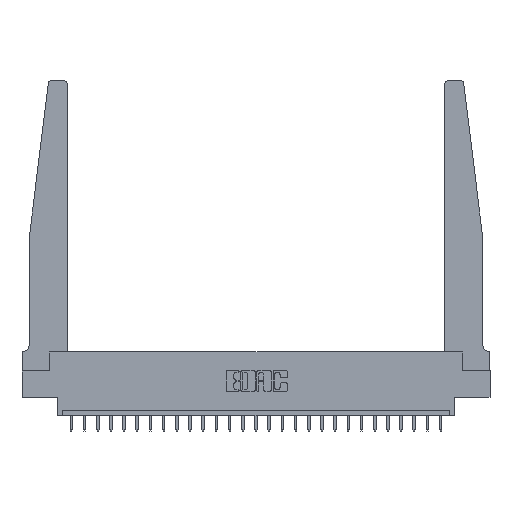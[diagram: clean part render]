
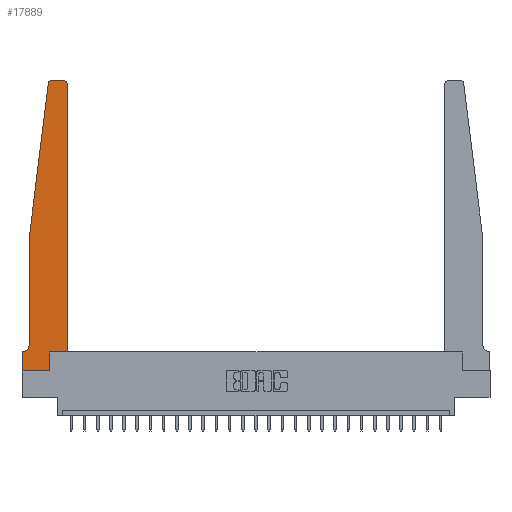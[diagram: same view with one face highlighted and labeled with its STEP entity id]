
A CAD part, top view. The second image highlights one B-rep face of the part: STEP entity #17889.
In plain terms, the highlighted planar face has unit normal (0, 0, 1).
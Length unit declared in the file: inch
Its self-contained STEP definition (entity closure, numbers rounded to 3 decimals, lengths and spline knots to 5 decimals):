
#10 = FACE_OUTER_BOUND ( 'NONE', #18840, .T. ) ;
#721 = DIRECTION ( 'NONE',  ( 0., -1., 0. ) ) ;
#957 = ORIENTED_EDGE ( 'NONE', *, *, #10690, .T. ) ;
#1084 = DIRECTION ( 'NONE',  ( 0., 1., 0. ) ) ;
#1565 = CARTESIAN_POINT ( 'NONE',  ( 0., 0.1875, 0.37 ) ) ;
#1606 = EDGE_CURVE ( 'NONE', #12865, #8407, #6839, .T. ) ;
#1644 = ORIENTED_EDGE ( 'NONE', *, *, #5036, .T. ) ;
#1809 = VERTEX_POINT ( 'NONE', #23196 ) ;
#2691 = ORIENTED_EDGE ( 'NONE', *, *, #24000, .T. ) ;
#2729 = DIRECTION ( 'NONE',  ( 0., 1., 0. ) ) ;
#2751 = VERTEX_POINT ( 'NONE', #13256 ) ;
#2815 = VERTEX_POINT ( 'NONE', #23662 ) ;
#3109 = ORIENTED_EDGE ( 'NONE', *, *, #23587, .T. ) ;
#3194 = VECTOR ( 'NONE', #2729, 39.37008 ) ;
#3248 = VERTEX_POINT ( 'NONE', #16357 ) ;
#3302 = AXIS2_PLACEMENT_3D ( 'NONE', #1565, #9700, #10102 ) ;
#3491 = AXIS2_PLACEMENT_3D ( 'NONE', #4339, #17725, #12045 ) ;
#3916 = ORIENTED_EDGE ( 'NONE', *, *, #8207, .T. ) ;
#3997 = VERTEX_POINT ( 'NONE', #21458 ) ;
#4089 = VERTEX_POINT ( 'NONE', #14762 ) ;
#4339 = CARTESIAN_POINT ( 'NONE',  ( 0.395, 2.72, 0.37 ) ) ;
#4904 = DIRECTION ( 'NONE',  ( 0., 0., -1. ) ) ;
#5036 = EDGE_CURVE ( 'NONE', #8407, #12965, #13755, .T. ) ;
#5824 = DIRECTION ( 'NONE',  ( 1., 0., 0. ) ) ;
#5901 = CARTESIAN_POINT ( 'NONE',  ( 0.27653, 2.72, 0.37 ) ) ;
#6569 = VECTOR ( 'NONE', #14403, 39.37008 ) ;
#6823 = DIRECTION ( 'NONE',  ( -1., 0., 0. ) ) ;
#6839 = CIRCLE ( 'NONE', #8254, 0.05 ) ;
#7009 = EDGE_CURVE ( 'NONE', #24431, #12865, #10088, .T. ) ;
#7024 = VECTOR ( 'NONE', #9410, 39.37008 ) ;
#7261 = VECTOR ( 'NONE', #1084, 39.37008 ) ;
#7342 = VERTEX_POINT ( 'NONE', #7566 ) ;
#7566 = CARTESIAN_POINT ( 'NONE',  ( 0., 0., 0.37 ) ) ;
#7690 = ORIENTED_EDGE ( 'NONE', *, *, #12557, .T. ) ;
#8207 = EDGE_CURVE ( 'NONE', #7342, #3248, #18680, .T. ) ;
#8254 = AXIS2_PLACEMENT_3D ( 'NONE', #16373, #4904, #6823 ) ;
#8407 = VERTEX_POINT ( 'NONE', #11729 ) ;
#8481 = LINE ( 'NONE', #8640, #7261 ) ;
#8640 = CARTESIAN_POINT ( 'NONE',  ( 0.2605, 0.18, 0.37 ) ) ;
#8898 = LINE ( 'NONE', #21751, #3194 ) ;
#9410 = DIRECTION ( 'NONE',  ( 1., 0., 0. ) ) ;
#9700 = DIRECTION ( 'NONE',  ( 0., 0., 1. ) ) ;
#9701 = VECTOR ( 'NONE', #11480, 39.37008 ) ;
#10005 = VECTOR ( 'NONE', #721, 39.37008 ) ;
#10060 = CIRCLE ( 'NONE', #15033, 0.03 ) ;
#10088 = LINE ( 'NONE', #23839, #14315 ) ;
#10102 = DIRECTION ( 'NONE',  ( 1., 0., 0. ) ) ;
#10339 = VECTOR ( 'NONE', #17485, 39.37008 ) ;
#10530 = EDGE_CURVE ( 'NONE', #1809, #2815, #8898, .T. ) ;
#10690 = EDGE_CURVE ( 'NONE', #3997, #23022, #14297, .T. ) ;
#11480 = DIRECTION ( 'NONE',  ( -0.122, -0.992, 0. ) ) ;
#11729 = CARTESIAN_POINT ( 'NONE',  ( 0.015, 0.1875, 0.37 ) ) ;
#11876 = CARTESIAN_POINT ( 'NONE',  ( 0.425, 0.18, 0.37 ) ) ;
#12045 = DIRECTION ( 'NONE',  ( 1., 0., 0. ) ) ;
#12557 = EDGE_CURVE ( 'NONE', #3248, #4089, #8481, .T. ) ;
#12865 = VERTEX_POINT ( 'NONE', #16001 ) ;
#12965 = VERTEX_POINT ( 'NONE', #21461 ) ;
#13154 = ORIENTED_EDGE ( 'NONE', *, *, #1606, .T. ) ;
#13256 = CARTESIAN_POINT ( 'NONE',  ( 0.24675, 2.72367, 0.37 ) ) ;
#13571 = LINE ( 'NONE', #21082, #9701 ) ;
#13755 = LINE ( 'NONE', #20115, #6569 ) ;
#14296 = CARTESIAN_POINT ( 'NONE',  ( 0., 0., 0.37 ) ) ;
#14297 = LINE ( 'NONE', #14437, #17247 ) ;
#14315 = VECTOR ( 'NONE', #19960, 39.37008 ) ;
#14403 = DIRECTION ( 'NONE',  ( -1., 0., 0. ) ) ;
#14437 = CARTESIAN_POINT ( 'NONE',  ( 0.25, 2.75, 0.37 ) ) ;
#14762 = CARTESIAN_POINT ( 'NONE',  ( 0.2605, 0.18, 0.37 ) ) ;
#15033 = AXIS2_PLACEMENT_3D ( 'NONE', #5901, #17303, #5824 ) ;
#15222 = ORIENTED_EDGE ( 'NONE', *, *, #19550, .T. ) ;
#15533 = EDGE_CURVE ( 'NONE', #2815, #3997, #17134, .T. ) ;
#16001 = CARTESIAN_POINT ( 'NONE',  ( 0.065, 0.2375, 0.37 ) ) ;
#16251 = ORIENTED_EDGE ( 'NONE', *, *, #20805, .T. ) ;
#16357 = CARTESIAN_POINT ( 'NONE',  ( 0.2605, 0., 0.37 ) ) ;
#16373 = CARTESIAN_POINT ( 'NONE',  ( 0.015, 0.2375, 0.37 ) ) ;
#16885 = LINE ( 'NONE', #14296, #10005 ) ;
#16929 = CARTESIAN_POINT ( 'NONE',  ( 0., 0., 0.37 ) ) ;
#17134 = CIRCLE ( 'NONE', #3491, 0.03 ) ;
#17247 = VECTOR ( 'NONE', #22078, 39.37008 ) ;
#17303 = DIRECTION ( 'NONE',  ( 0., 0., 1. ) ) ;
#17485 = DIRECTION ( 'NONE',  ( 1., 0., 0. ) ) ;
#17656 = CARTESIAN_POINT ( 'NONE',  ( 0.27653, 2.75, 0.37 ) ) ;
#17725 = DIRECTION ( 'NONE',  ( 0., 0., 1. ) ) ;
#17889 = ADVANCED_FACE ( 'NONE', ( #10 ), #23643, .T. ) ;
#18335 = ORIENTED_EDGE ( 'NONE', *, *, #15533, .T. ) ;
#18346 = ORIENTED_EDGE ( 'NONE', *, *, #10530, .T. ) ;
#18680 = LINE ( 'NONE', #16929, #7024 ) ;
#18840 = EDGE_LOOP ( 'NONE', ( #957, #15222, #2691, #22019, #13154, #1644, #3109, #3916, #7690, #16251, #18346, #18335 ) ) ;
#19550 = EDGE_CURVE ( 'NONE', #23022, #2751, #10060, .T. ) ;
#19882 = LINE ( 'NONE', #11876, #10339 ) ;
#19960 = DIRECTION ( 'NONE',  ( 0., -1., 0. ) ) ;
#20115 = CARTESIAN_POINT ( 'NONE',  ( 0.065, 0.1875, 0.37 ) ) ;
#20805 = EDGE_CURVE ( 'NONE', #4089, #1809, #19882, .T. ) ;
#21082 = CARTESIAN_POINT ( 'NONE',  ( 0.065, 1.25, 0.37 ) ) ;
#21458 = CARTESIAN_POINT ( 'NONE',  ( 0.395, 2.75, 0.37 ) ) ;
#21461 = CARTESIAN_POINT ( 'NONE',  ( 0., 0.1875, 0.37 ) ) ;
#21478 = CARTESIAN_POINT ( 'NONE',  ( 0.065, 1.25, 0.37 ) ) ;
#21751 = CARTESIAN_POINT ( 'NONE',  ( 0.425, 0.18, 0.37 ) ) ;
#22019 = ORIENTED_EDGE ( 'NONE', *, *, #7009, .T. ) ;
#22078 = DIRECTION ( 'NONE',  ( -1., 0., 0. ) ) ;
#23022 = VERTEX_POINT ( 'NONE', #17656 ) ;
#23196 = CARTESIAN_POINT ( 'NONE',  ( 0.425, 0.18, 0.37 ) ) ;
#23587 = EDGE_CURVE ( 'NONE', #12965, #7342, #16885, .T. ) ;
#23643 = PLANE ( 'NONE',  #3302 ) ;
#23662 = CARTESIAN_POINT ( 'NONE',  ( 0.425, 2.72, 0.37 ) ) ;
#23839 = CARTESIAN_POINT ( 'NONE',  ( 0.065, 1.25, 0.37 ) ) ;
#24000 = EDGE_CURVE ( 'NONE', #2751, #24431, #13571, .T. ) ;
#24431 = VERTEX_POINT ( 'NONE', #21478 ) ;
